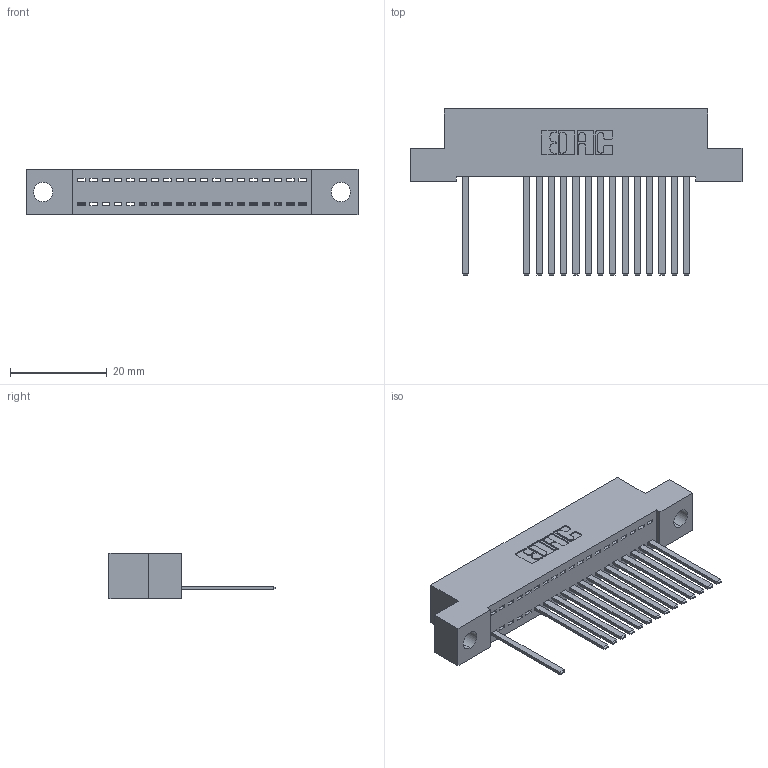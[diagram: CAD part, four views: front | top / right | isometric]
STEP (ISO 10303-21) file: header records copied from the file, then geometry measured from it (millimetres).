
FILE_DESCRIPTION (( 'STEP AP203' ), '1' );
FILE_NAME ('392-019-544-104.STEP', '2018-08-15T05:37:50', ( '' ), ( '' ), 'SwSTEP 2.0', 'SolidWorks 2016', '' );
FILE_SCHEMA (( 'CONFIG_CONTROL_DESIGN' ));
Length unit declared in the file: inch
Products named in the file (3): 342 Part_.156 TH; 345-292-001_345-293-144; 392-019-544-104
Assembly tree (16 placements, depth 2):
  392-019-544-104
    342 Part_.156 TH
    345-292-001_345-293-144  x15
Bounding box: 68.58 x 34.3 x 9.4 mm (x, y, z)
Volume: 5969.3 mm3; surface area: 8412.4 mm2
Topology: 16 solids, 16 shells, 938 faces, 2837 edges, 1870 vertices
Faces by surface type: plane 684, cylinder 254
Entity records: 14149 total; most frequent: CARTESIAN_POINT 2467, ORIENTED_EDGE 2426, DIRECTION 2119, EDGE_CURVE 1213, VECTOR 1089, LINE 1089, VERTEX_POINT 806, AXIS2_PLACEMENT_3D 515
